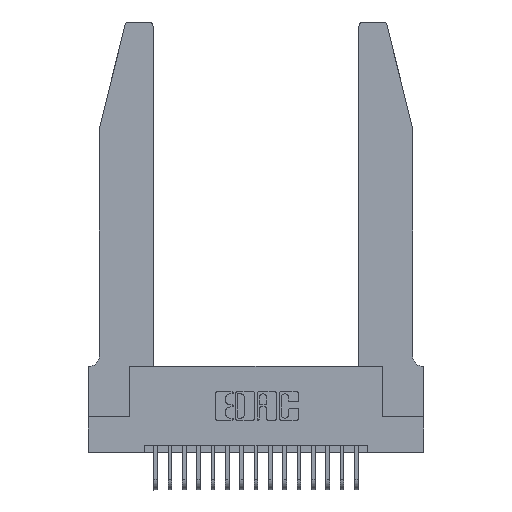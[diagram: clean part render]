
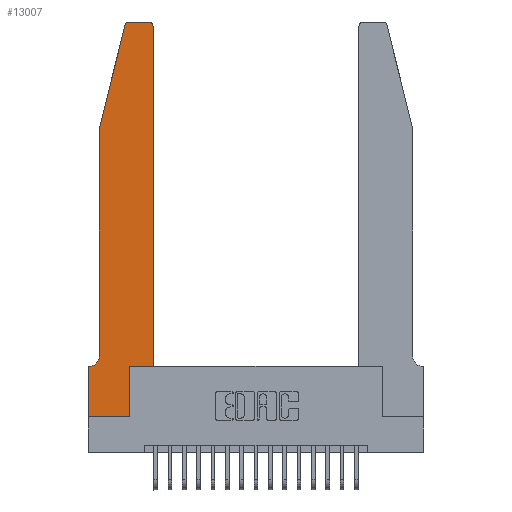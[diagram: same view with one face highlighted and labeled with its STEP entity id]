
A CAD part, top view. The second image highlights one B-rep face of the part: STEP entity #13007.
In plain terms, the highlighted planar face has unit normal (0, 0, 1).
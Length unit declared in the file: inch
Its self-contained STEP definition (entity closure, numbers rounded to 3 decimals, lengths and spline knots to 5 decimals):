
#544 = EDGE_CURVE ( 'NONE', #5024, #6005, #17838, .T. ) ;
#654 = LINE ( 'NONE', #13491, #19006 ) ;
#832 = CARTESIAN_POINT ( 'NONE',  ( 0., 0.35, 0.37 ) ) ;
#1345 = VECTOR ( 'NONE', #6719, 39.37008 ) ;
#1528 = DIRECTION ( 'NONE',  ( 0., 1., 0. ) ) ;
#1732 = CARTESIAN_POINT ( 'NONE',  ( 0.2865, 0.35, 0.37 ) ) ;
#1909 = CARTESIAN_POINT ( 'NONE',  ( 0.0055, 0.42, 0.37 ) ) ;
#2030 = ORIENTED_EDGE ( 'NONE', *, *, #14470, .T. ) ;
#2285 = EDGE_CURVE ( 'NONE', #11688, #7268, #11249, .T. ) ;
#2418 = CARTESIAN_POINT ( 'NONE',  ( 0.4505, 2.72, 0.37 ) ) ;
#2622 = CARTESIAN_POINT ( 'NONE',  ( 0.0055, 0.35, 0.37 ) ) ;
#2936 = EDGE_CURVE ( 'NONE', #4406, #8603, #18016, .T. ) ;
#3251 = CARTESIAN_POINT ( 'NONE',  ( 0., 0., 0.37 ) ) ;
#3501 = DIRECTION ( 'NONE',  ( -1., 0., 0. ) ) ;
#3897 = VECTOR ( 'NONE', #4827, 39.37008 ) ;
#3990 = CARTESIAN_POINT ( 'NONE',  ( 0.284, 2.72, 0.37 ) ) ;
#4406 = VERTEX_POINT ( 'NONE', #2418 ) ;
#4661 = VECTOR ( 'NONE', #11768, 39.37008 ) ;
#4827 = DIRECTION ( 'NONE',  ( 1., 0., 0. ) ) ;
#4983 = ORIENTED_EDGE ( 'NONE', *, *, #5658, .T. ) ;
#5024 = VERTEX_POINT ( 'NONE', #5482 ) ;
#5038 = CARTESIAN_POINT ( 'NONE',  ( 0.0755, 2., 0.37 ) ) ;
#5139 = CARTESIAN_POINT ( 'NONE',  ( 0., 0., 0.37 ) ) ;
#5482 = CARTESIAN_POINT ( 'NONE',  ( 0.2865, 0., 0.37 ) ) ;
#5575 = DIRECTION ( 'NONE',  ( 1., 0., 0. ) ) ;
#5658 = EDGE_CURVE ( 'NONE', #7268, #17027, #16766, .T. ) ;
#5749 = VERTEX_POINT ( 'NONE', #13439 ) ;
#5754 = AXIS2_PLACEMENT_3D ( 'NONE', #9097, #19583, #10609 ) ;
#5822 = VECTOR ( 'NONE', #1528, 39.37008 ) ;
#5935 = EDGE_CURVE ( 'NONE', #5749, #5024, #15995, .T. ) ;
#6005 = VERTEX_POINT ( 'NONE', #1732 ) ;
#6052 = LINE ( 'NONE', #5139, #1345 ) ;
#6058 = LINE ( 'NONE', #7956, #13561 ) ;
#6583 = ORIENTED_EDGE ( 'NONE', *, *, #544, .T. ) ;
#6719 = DIRECTION ( 'NONE',  ( 0., -1., 0. ) ) ;
#6758 = VECTOR ( 'NONE', #10089, 39.37008 ) ;
#7268 = VERTEX_POINT ( 'NONE', #17930 ) ;
#7348 = CARTESIAN_POINT ( 'NONE',  ( 0.4505, 0.35, 0.37 ) ) ;
#7376 = VERTEX_POINT ( 'NONE', #9197 ) ;
#7448 = ORIENTED_EDGE ( 'NONE', *, *, #5935, .T. ) ;
#7485 = EDGE_CURVE ( 'NONE', #6005, #8053, #6058, .T. ) ;
#7956 = CARTESIAN_POINT ( 'NONE',  ( 0.4505, 0.35, 0.37 ) ) ;
#7965 = VERTEX_POINT ( 'NONE', #14658 ) ;
#8053 = VERTEX_POINT ( 'NONE', #7348 ) ;
#8055 = CARTESIAN_POINT ( 'NONE',  ( 0.2605, 2.75, 0.37 ) ) ;
#8603 = VERTEX_POINT ( 'NONE', #19309 ) ;
#9003 = ORIENTED_EDGE ( 'NONE', *, *, #2936, .T. ) ;
#9097 = CARTESIAN_POINT ( 'NONE',  ( 0.4205, 2.72, 0.37 ) ) ;
#9197 = CARTESIAN_POINT ( 'NONE',  ( 0.284, 2.75, 0.37 ) ) ;
#9448 = DIRECTION ( 'NONE',  ( 1., 0., 0. ) ) ;
#9756 = EDGE_CURVE ( 'NONE', #7376, #11688, #17749, .T. ) ;
#10022 = AXIS2_PLACEMENT_3D ( 'NONE', #1909, #12616, #3501 ) ;
#10027 = EDGE_CURVE ( 'NONE', #17027, #16463, #13032, .T. ) ;
#10089 = DIRECTION ( 'NONE',  ( -0.239, -0.971, 0. ) ) ;
#10162 = DIRECTION ( 'NONE',  ( 1., 0., 0. ) ) ;
#10249 = CARTESIAN_POINT ( 'NONE',  ( 0.0755, 2., 0.37 ) ) ;
#10352 = DIRECTION ( 'NONE',  ( -1., 0., 0. ) ) ;
#10396 = AXIS2_PLACEMENT_3D ( 'NONE', #3990, #14590, #5575 ) ;
#10609 = DIRECTION ( 'NONE',  ( 1., 0., 0. ) ) ;
#10709 = ORIENTED_EDGE ( 'NONE', *, *, #2285, .T. ) ;
#11003 = CARTESIAN_POINT ( 'NONE',  ( 0.2865, 0.35, 0.37 ) ) ;
#11015 = VECTOR ( 'NONE', #18514, 39.37008 ) ;
#11249 = LINE ( 'NONE', #5038, #6758 ) ;
#11515 = EDGE_LOOP ( 'NONE', ( #17158, #19149, #10709, #4983, #13575, #13959, #2030, #7448, #6583, #14945, #13191, #9003 ) ) ;
#11688 = VERTEX_POINT ( 'NONE', #18849 ) ;
#11768 = DIRECTION ( 'NONE',  ( 0., -1., 0. ) ) ;
#12616 = DIRECTION ( 'NONE',  ( 0., 0., -1. ) ) ;
#13007 = ADVANCED_FACE ( 'NONE', ( #18321 ), #16147, .T. ) ;
#13032 = CIRCLE ( 'NONE', #10022, 0.07 ) ;
#13191 = ORIENTED_EDGE ( 'NONE', *, *, #13618, .T. ) ;
#13343 = CARTESIAN_POINT ( 'NONE',  ( 0.0755, 0.35, 0.37 ) ) ;
#13439 = CARTESIAN_POINT ( 'NONE',  ( 0., 0., 0.37 ) ) ;
#13491 = CARTESIAN_POINT ( 'NONE',  ( 0.4505, 0.35, 0.37 ) ) ;
#13561 = VECTOR ( 'NONE', #9448, 39.37008 ) ;
#13575 = ORIENTED_EDGE ( 'NONE', *, *, #10027, .T. ) ;
#13618 = EDGE_CURVE ( 'NONE', #8053, #4406, #654, .T. ) ;
#13626 = DIRECTION ( 'NONE',  ( 0., 1., 0. ) ) ;
#13959 = ORIENTED_EDGE ( 'NONE', *, *, #17004, .T. ) ;
#14403 = EDGE_CURVE ( 'NONE', #8603, #7376, #18961, .T. ) ;
#14470 = EDGE_CURVE ( 'NONE', #7965, #5749, #6052, .T. ) ;
#14590 = DIRECTION ( 'NONE',  ( 0., 0., 1. ) ) ;
#14658 = CARTESIAN_POINT ( 'NONE',  ( 0., 0.35, 0.37 ) ) ;
#14945 = ORIENTED_EDGE ( 'NONE', *, *, #7485, .T. ) ;
#15850 = VECTOR ( 'NONE', #10352, 39.37008 ) ;
#15995 = LINE ( 'NONE', #3251, #3897 ) ;
#16147 = PLANE ( 'NONE',  #19646 ) ;
#16463 = VERTEX_POINT ( 'NONE', #2622 ) ;
#16480 = CARTESIAN_POINT ( 'NONE',  ( 0.0755, 0.42, 0.37 ) ) ;
#16766 = LINE ( 'NONE', #10249, #4661 ) ;
#17004 = EDGE_CURVE ( 'NONE', #16463, #7965, #19366, .T. ) ;
#17027 = VERTEX_POINT ( 'NONE', #16480 ) ;
#17158 = ORIENTED_EDGE ( 'NONE', *, *, #14403, .T. ) ;
#17749 = CIRCLE ( 'NONE', #10396, 0.03 ) ;
#17838 = LINE ( 'NONE', #11003, #5822 ) ;
#17930 = CARTESIAN_POINT ( 'NONE',  ( 0.0755, 2., 0.37 ) ) ;
#18016 = CIRCLE ( 'NONE', #5754, 0.03 ) ;
#18321 = FACE_OUTER_BOUND ( 'NONE', #11515, .T. ) ;
#18514 = DIRECTION ( 'NONE',  ( -1., 0., 0. ) ) ;
#18849 = CARTESIAN_POINT ( 'NONE',  ( 0.25487, 2.72718, 0.37 ) ) ;
#18961 = LINE ( 'NONE', #8055, #11015 ) ;
#19006 = VECTOR ( 'NONE', #13626, 39.37008 ) ;
#19135 = DIRECTION ( 'NONE',  ( 0., 0., 1. ) ) ;
#19149 = ORIENTED_EDGE ( 'NONE', *, *, #9756, .T. ) ;
#19309 = CARTESIAN_POINT ( 'NONE',  ( 0.4205, 2.75, 0.37 ) ) ;
#19366 = LINE ( 'NONE', #13343, #15850 ) ;
#19583 = DIRECTION ( 'NONE',  ( 0., 0., 1. ) ) ;
#19646 = AXIS2_PLACEMENT_3D ( 'NONE', #832, #19135, #10162 ) ;
